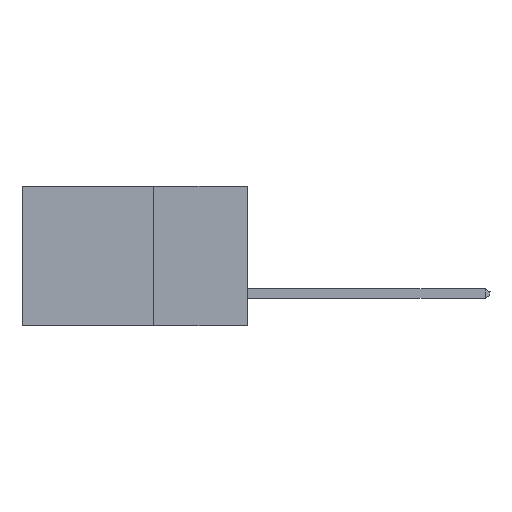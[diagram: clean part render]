
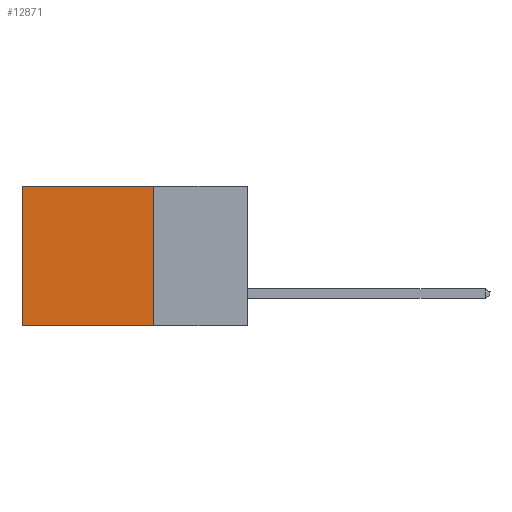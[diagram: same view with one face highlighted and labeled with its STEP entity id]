
A CAD part, left-side view. The second image highlights one B-rep face of the part: STEP entity #12871.
In plain terms, the highlighted planar face has unit normal (-1, 0, 0).
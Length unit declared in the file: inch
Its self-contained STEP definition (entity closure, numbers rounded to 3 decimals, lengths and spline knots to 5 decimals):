
#431 = EDGE_CURVE ( 'NONE', #2739, #12101, #7674, .T. ) ;
#534 = CARTESIAN_POINT ( 'NONE',  ( 0.2615, 0.25, 0. ) ) ;
#959 = LINE ( 'NONE', #10016, #9806 ) ;
#1284 = ORIENTED_EDGE ( 'NONE', *, *, #431, .F. ) ;
#1658 = VERTEX_POINT ( 'NONE', #2897 ) ;
#1781 = VECTOR ( 'NONE', #9052, 39.37008 ) ;
#1891 = EDGE_CURVE ( 'NONE', #5690, #1658, #8034, .T. ) ;
#2514 = CARTESIAN_POINT ( 'NONE',  ( 0.2615, 0.6, -0.37 ) ) ;
#2739 = VERTEX_POINT ( 'NONE', #534 ) ;
#2893 = DIRECTION ( 'NONE',  ( 1., 0., 0. ) ) ;
#2897 = CARTESIAN_POINT ( 'NONE',  ( 0.2615, 0.6, -0.37 ) ) ;
#3172 = CARTESIAN_POINT ( 'NONE',  ( 0.2615, 0.25, -0.37 ) ) ;
#3321 = AXIS2_PLACEMENT_3D ( 'NONE', #12892, #2893, #5069 ) ;
#3981 = PLANE ( 'NONE',  #3321 ) ;
#4151 = CARTESIAN_POINT ( 'NONE',  ( 0.2615, 0.25, -0.37 ) ) ;
#5069 = DIRECTION ( 'NONE',  ( 0., 0., -1. ) ) ;
#5148 = DIRECTION ( 'NONE',  ( 0., 1., 0. ) ) ;
#5690 = VERTEX_POINT ( 'NONE', #7169 ) ;
#5773 = ORIENTED_EDGE ( 'NONE', *, *, #12593, .F. ) ;
#6758 = EDGE_CURVE ( 'NONE', #2739, #5690, #7470, .T. ) ;
#7024 = EDGE_LOOP ( 'NONE', ( #14347, #5773, #1284, #10410 ) ) ;
#7169 = CARTESIAN_POINT ( 'NONE',  ( 0.2615, 0.6, 0. ) ) ;
#7470 = LINE ( 'NONE', #11924, #10013 ) ;
#7674 = LINE ( 'NONE', #3172, #13725 ) ;
#8034 = LINE ( 'NONE', #2514, #1781 ) ;
#8841 = DIRECTION ( 'NONE',  ( 0., 0., -1. ) ) ;
#9052 = DIRECTION ( 'NONE',  ( 0., 0., -1. ) ) ;
#9806 = VECTOR ( 'NONE', #14209, 39.37008 ) ;
#10013 = VECTOR ( 'NONE', #5148, 39.37008 ) ;
#10016 = CARTESIAN_POINT ( 'NONE',  ( 0.2615, 0.25, -0.37 ) ) ;
#10410 = ORIENTED_EDGE ( 'NONE', *, *, #6758, .T. ) ;
#11924 = CARTESIAN_POINT ( 'NONE',  ( 0.2615, 0.25, 0. ) ) ;
#12101 = VERTEX_POINT ( 'NONE', #4151 ) ;
#12593 = EDGE_CURVE ( 'NONE', #12101, #1658, #959, .T. ) ;
#12871 = ADVANCED_FACE ( 'NONE', ( #12958 ), #3981, .F. ) ;
#12892 = CARTESIAN_POINT ( 'NONE',  ( 0.2615, 0.25, -0.37 ) ) ;
#12958 = FACE_OUTER_BOUND ( 'NONE', #7024, .T. ) ;
#13725 = VECTOR ( 'NONE', #8841, 39.37008 ) ;
#14209 = DIRECTION ( 'NONE',  ( 0., 1., 0. ) ) ;
#14347 = ORIENTED_EDGE ( 'NONE', *, *, #1891, .T. ) ;
